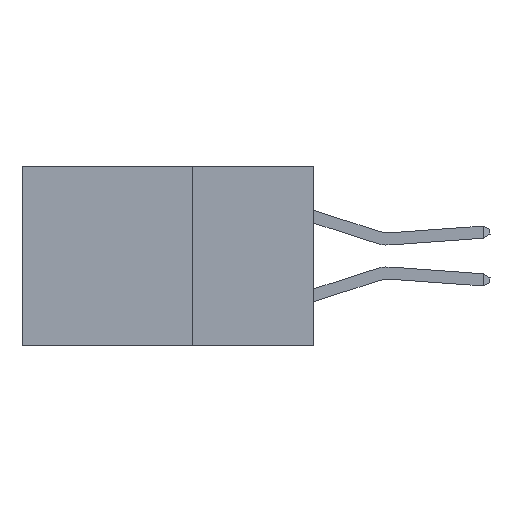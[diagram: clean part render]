
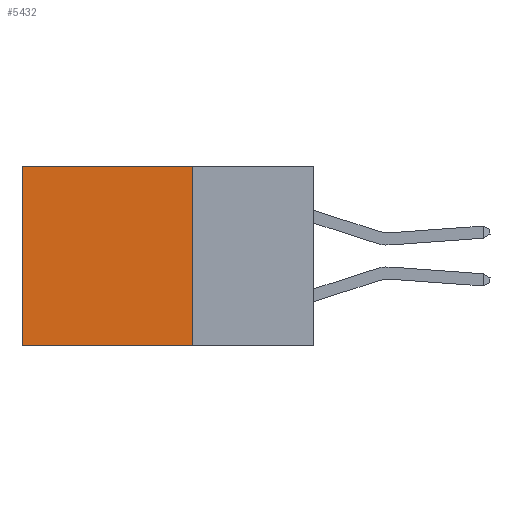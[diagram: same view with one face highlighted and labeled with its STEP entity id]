
A CAD part, left-side view. The second image highlights one B-rep face of the part: STEP entity #5432.
In plain terms, the highlighted planar face has unit normal (-1, 0, 0).
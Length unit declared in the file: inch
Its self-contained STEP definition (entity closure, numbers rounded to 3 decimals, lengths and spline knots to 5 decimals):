
#215 = VERTEX_POINT ( 'NONE', #11361 ) ;
#2003 = EDGE_LOOP ( 'NONE', ( #4217, #4182, #15993, #17363 ) ) ;
#2218 = VERTEX_POINT ( 'NONE', #9843 ) ;
#2288 = VERTEX_POINT ( 'NONE', #16202 ) ;
#2433 = CARTESIAN_POINT ( 'NONE',  ( 0.2875, 0.25, -0.37 ) ) ;
#3232 = LINE ( 'NONE', #17379, #7024 ) ;
#4158 = AXIS2_PLACEMENT_3D ( 'NONE', #11818, #14818, #5364 ) ;
#4182 = ORIENTED_EDGE ( 'NONE', *, *, #20277, .F. ) ;
#4217 = ORIENTED_EDGE ( 'NONE', *, *, #15986, .T. ) ;
#5364 = DIRECTION ( 'NONE',  ( 0., 0., -1. ) ) ;
#5432 = ADVANCED_FACE ( 'NONE', ( #10859 ), #10225, .F. ) ;
#7024 = VECTOR ( 'NONE', #11034, 39.37008 ) ;
#7344 = VECTOR ( 'NONE', #18899, 39.37008 ) ;
#7524 = CARTESIAN_POINT ( 'NONE',  ( 0.2875, 0.6, 0. ) ) ;
#8013 = DIRECTION ( 'NONE',  ( 0., 1., 0. ) ) ;
#8219 = CARTESIAN_POINT ( 'NONE',  ( 0.2875, 0.25, -0.37 ) ) ;
#9035 = EDGE_CURVE ( 'NONE', #2218, #215, #3232, .T. ) ;
#9843 = CARTESIAN_POINT ( 'NONE',  ( 0.2875, 0.25, 0. ) ) ;
#10225 = PLANE ( 'NONE',  #4158 ) ;
#10859 = FACE_OUTER_BOUND ( 'NONE', #2003, .T. ) ;
#11034 = DIRECTION ( 'NONE',  ( 0., 1., 0. ) ) ;
#11361 = CARTESIAN_POINT ( 'NONE',  ( 0.2875, 0.6, 0. ) ) ;
#11477 = EDGE_CURVE ( 'NONE', #2218, #13518, #12270, .T. ) ;
#11818 = CARTESIAN_POINT ( 'NONE',  ( 0.2875, 0.25, 0. ) ) ;
#12270 = LINE ( 'NONE', #12362, #7344 ) ;
#12362 = CARTESIAN_POINT ( 'NONE',  ( 0.2875, 0.25, 0. ) ) ;
#12604 = LINE ( 'NONE', #2433, #13090 ) ;
#13090 = VECTOR ( 'NONE', #8013, 39.37008 ) ;
#13518 = VERTEX_POINT ( 'NONE', #8219 ) ;
#13594 = VECTOR ( 'NONE', #20131, 39.37008 ) ;
#14097 = LINE ( 'NONE', #7524, #13594 ) ;
#14818 = DIRECTION ( 'NONE',  ( 1., 0., 0. ) ) ;
#15986 = EDGE_CURVE ( 'NONE', #215, #2288, #14097, .T. ) ;
#15993 = ORIENTED_EDGE ( 'NONE', *, *, #11477, .F. ) ;
#16202 = CARTESIAN_POINT ( 'NONE',  ( 0.2875, 0.6, -0.37 ) ) ;
#17363 = ORIENTED_EDGE ( 'NONE', *, *, #9035, .T. ) ;
#17379 = CARTESIAN_POINT ( 'NONE',  ( 0.2875, 0.25, 0. ) ) ;
#18899 = DIRECTION ( 'NONE',  ( 0., 0., -1. ) ) ;
#20131 = DIRECTION ( 'NONE',  ( 0., 0., -1. ) ) ;
#20277 = EDGE_CURVE ( 'NONE', #13518, #2288, #12604, .T. ) ;
